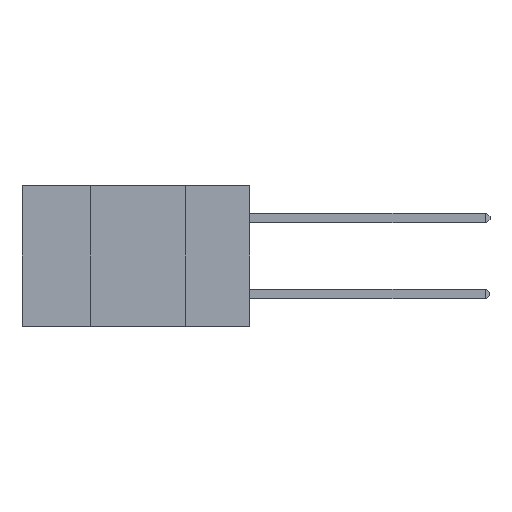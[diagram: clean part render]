
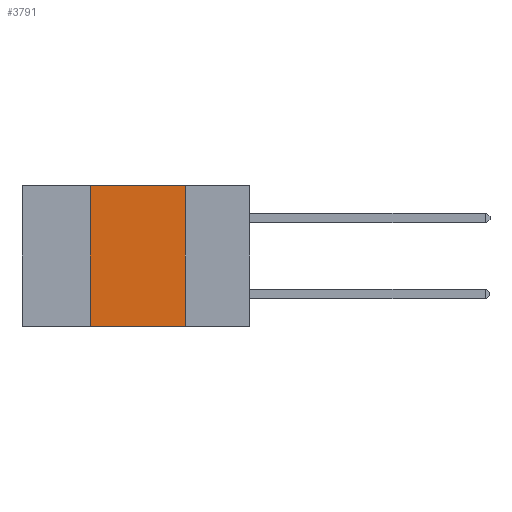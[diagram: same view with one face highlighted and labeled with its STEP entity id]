
A CAD part, left-side view. The second image highlights one B-rep face of the part: STEP entity #3791.
In plain terms, the highlighted planar face has unit normal (-1, 0, 0).
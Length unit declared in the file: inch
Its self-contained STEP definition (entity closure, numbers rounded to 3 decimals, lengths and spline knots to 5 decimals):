
#788 = DIRECTION ( 'NONE',  ( 0., 0., -1. ) ) ;
#1737 = CARTESIAN_POINT ( 'NONE',  ( 0., 0.42, -0.37 ) ) ;
#1882 = DIRECTION ( 'NONE',  ( 0., 0., 1. ) ) ;
#2533 = ORIENTED_EDGE ( 'NONE', *, *, #11728, .F. ) ;
#3791 = ADVANCED_FACE ( 'NONE', ( #11519 ), #16755, .F. ) ;
#4766 = ORIENTED_EDGE ( 'NONE', *, *, #15914, .F. ) ;
#5116 = VECTOR ( 'NONE', #18510, 39.37008 ) ;
#5880 = ORIENTED_EDGE ( 'NONE', *, *, #12170, .T. ) ;
#6068 = LINE ( 'NONE', #17305, #6530 ) ;
#6097 = CARTESIAN_POINT ( 'NONE',  ( 0., 0.17, -0.37 ) ) ;
#6530 = VECTOR ( 'NONE', #7298, 39.37008 ) ;
#6727 = VERTEX_POINT ( 'NONE', #1737 ) ;
#7226 = CARTESIAN_POINT ( 'NONE',  ( 0., 0.6, -0.37 ) ) ;
#7298 = DIRECTION ( 'NONE',  ( 0., -1., 0. ) ) ;
#7911 = AXIS2_PLACEMENT_3D ( 'NONE', #15200, #17140, #788 ) ;
#8415 = EDGE_CURVE ( 'NONE', #14064, #16055, #6068, .T. ) ;
#8502 = VECTOR ( 'NONE', #9124, 39.37008 ) ;
#8723 = CARTESIAN_POINT ( 'NONE',  ( 0., 0.42, 0. ) ) ;
#9124 = DIRECTION ( 'NONE',  ( 0., 0., -1. ) ) ;
#10136 = EDGE_LOOP ( 'NONE', ( #2533, #16507, #4766, #5880 ) ) ;
#10905 = CARTESIAN_POINT ( 'NONE',  ( 0., 0.42, 0. ) ) ;
#11519 = FACE_OUTER_BOUND ( 'NONE', #10136, .T. ) ;
#11687 = LINE ( 'NONE', #10905, #15833 ) ;
#11728 = EDGE_CURVE ( 'NONE', #16055, #18488, #17999, .T. ) ;
#12170 = EDGE_CURVE ( 'NONE', #6727, #18488, #16190, .T. ) ;
#14002 = CARTESIAN_POINT ( 'NONE',  ( 0., 0.17, 0. ) ) ;
#14064 = VERTEX_POINT ( 'NONE', #8723 ) ;
#14899 = CARTESIAN_POINT ( 'NONE',  ( 0., 0.17, 0. ) ) ;
#15200 = CARTESIAN_POINT ( 'NONE',  ( 0., 0.6, 0. ) ) ;
#15833 = VECTOR ( 'NONE', #1882, 39.37008 ) ;
#15914 = EDGE_CURVE ( 'NONE', #6727, #14064, #11687, .T. ) ;
#16055 = VERTEX_POINT ( 'NONE', #14002 ) ;
#16190 = LINE ( 'NONE', #7226, #5116 ) ;
#16507 = ORIENTED_EDGE ( 'NONE', *, *, #8415, .F. ) ;
#16755 = PLANE ( 'NONE',  #7911 ) ;
#17140 = DIRECTION ( 'NONE',  ( 1., 0., 0. ) ) ;
#17305 = CARTESIAN_POINT ( 'NONE',  ( 0., 0.6, 0. ) ) ;
#17999 = LINE ( 'NONE', #14899, #8502 ) ;
#18488 = VERTEX_POINT ( 'NONE', #6097 ) ;
#18510 = DIRECTION ( 'NONE',  ( 0., -1., 0. ) ) ;
